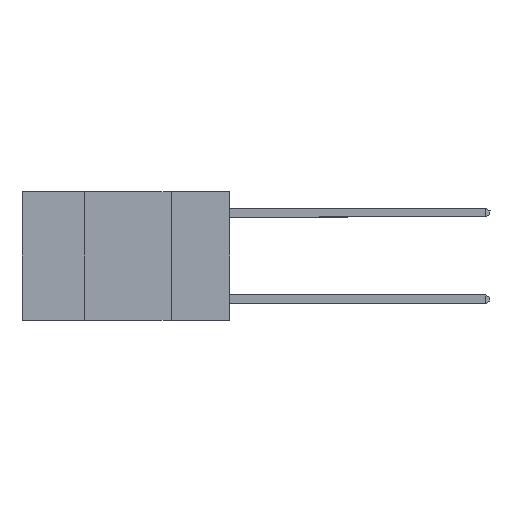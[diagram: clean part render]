
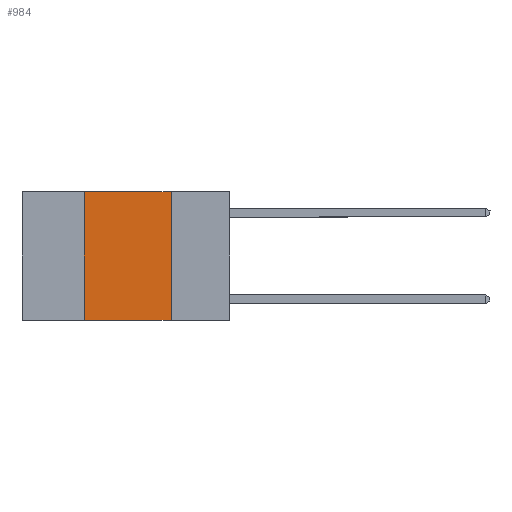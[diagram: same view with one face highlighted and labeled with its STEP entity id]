
A CAD part, left-side view. The second image highlights one B-rep face of the part: STEP entity #984.
In plain terms, the highlighted planar face has unit normal (-1, 0, 0).
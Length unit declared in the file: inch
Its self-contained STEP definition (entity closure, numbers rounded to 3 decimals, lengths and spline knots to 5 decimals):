
#164 = EDGE_CURVE ( 'NONE', #8033, #1645, #6122, .T. ) ;
#264 = VERTEX_POINT ( 'NONE', #8753 ) ;
#294 = CARTESIAN_POINT ( 'NONE',  ( 0., 0.17, 0. ) ) ;
#668 = LINE ( 'NONE', #6173, #2432 ) ;
#679 = EDGE_CURVE ( 'NONE', #8033, #264, #8008, .T. ) ;
#932 = VECTOR ( 'NONE', #3379, 39.37008 ) ;
#984 = ADVANCED_FACE ( 'NONE', ( #5897 ), #2350, .F. ) ;
#1017 = ORIENTED_EDGE ( 'NONE', *, *, #1222, .F. ) ;
#1222 = EDGE_CURVE ( 'NONE', #8291, #1645, #2430, .T. ) ;
#1311 = ORIENTED_EDGE ( 'NONE', *, *, #679, .F. ) ;
#1465 = CARTESIAN_POINT ( 'NONE',  ( 0., 0.17, 0. ) ) ;
#1622 = ORIENTED_EDGE ( 'NONE', *, *, #5111, .F. ) ;
#1645 = VERTEX_POINT ( 'NONE', #2452 ) ;
#2196 = ORIENTED_EDGE ( 'NONE', *, *, #164, .T. ) ;
#2246 = DIRECTION ( 'NONE',  ( 0., 0., -1. ) ) ;
#2350 = PLANE ( 'NONE',  #9134 ) ;
#2430 = LINE ( 'NONE', #1465, #6102 ) ;
#2432 = VECTOR ( 'NONE', #8324, 39.37008 ) ;
#2452 = CARTESIAN_POINT ( 'NONE',  ( 0., 0.17, -0.37 ) ) ;
#2551 = CARTESIAN_POINT ( 'NONE',  ( 0., 0.6, 0. ) ) ;
#2959 = EDGE_LOOP ( 'NONE', ( #1017, #1622, #1311, #2196 ) ) ;
#3379 = DIRECTION ( 'NONE',  ( 0., 0., 1. ) ) ;
#5111 = EDGE_CURVE ( 'NONE', #264, #8291, #668, .T. ) ;
#5897 = FACE_OUTER_BOUND ( 'NONE', #2959, .T. ) ;
#6102 = VECTOR ( 'NONE', #9179, 39.37008 ) ;
#6122 = LINE ( 'NONE', #7548, #8013 ) ;
#6173 = CARTESIAN_POINT ( 'NONE',  ( 0., 0.6, 0. ) ) ;
#6294 = CARTESIAN_POINT ( 'NONE',  ( 0., 0.42, 0. ) ) ;
#6395 = DIRECTION ( 'NONE',  ( 0., -1., 0. ) ) ;
#6536 = CARTESIAN_POINT ( 'NONE',  ( 0., 0.42, -0.37 ) ) ;
#7548 = CARTESIAN_POINT ( 'NONE',  ( 0., 0.6, -0.37 ) ) ;
#8008 = LINE ( 'NONE', #6294, #932 ) ;
#8013 = VECTOR ( 'NONE', #6395, 39.37008 ) ;
#8033 = VERTEX_POINT ( 'NONE', #6536 ) ;
#8291 = VERTEX_POINT ( 'NONE', #294 ) ;
#8324 = DIRECTION ( 'NONE',  ( 0., -1., 0. ) ) ;
#8433 = DIRECTION ( 'NONE',  ( 1., 0., 0. ) ) ;
#8753 = CARTESIAN_POINT ( 'NONE',  ( 0., 0.42, 0. ) ) ;
#9134 = AXIS2_PLACEMENT_3D ( 'NONE', #2551, #8433, #2246 ) ;
#9179 = DIRECTION ( 'NONE',  ( 0., 0., -1. ) ) ;
